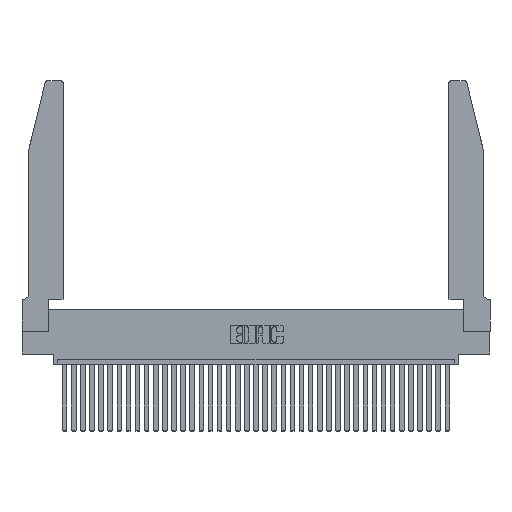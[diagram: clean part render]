
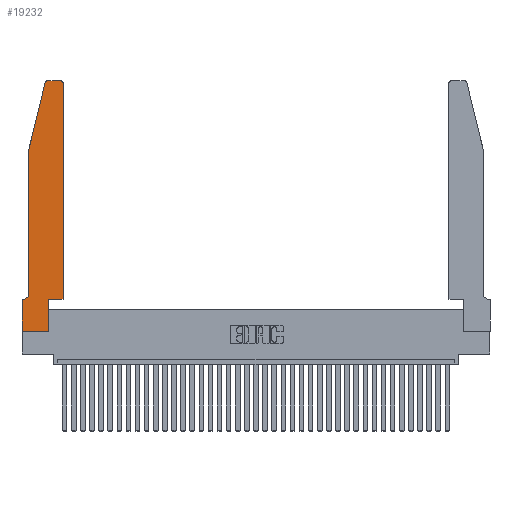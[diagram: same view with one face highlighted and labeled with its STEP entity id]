
A CAD part, top view. The second image highlights one B-rep face of the part: STEP entity #19232.
In plain terms, the highlighted planar face has unit normal (0, 0, 1).
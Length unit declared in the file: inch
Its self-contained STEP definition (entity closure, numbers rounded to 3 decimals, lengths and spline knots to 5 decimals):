
#397 = VERTEX_POINT ( 'NONE', #5148 ) ;
#623 = EDGE_CURVE ( 'NONE', #397, #15735, #32254, .T. ) ;
#2155 = FACE_OUTER_BOUND ( 'NONE', #23706, .T. ) ;
#2720 = DIRECTION ( 'NONE',  ( 0., 0., 1. ) ) ;
#2978 = VERTEX_POINT ( 'NONE', #31135 ) ;
#3154 = EDGE_CURVE ( 'NONE', #24123, #29250, #25392, .T. ) ;
#3217 = ORIENTED_EDGE ( 'NONE', *, *, #3154, .T. ) ;
#3383 = AXIS2_PLACEMENT_3D ( 'NONE', #30027, #23879, #4256 ) ;
#3392 = ORIENTED_EDGE ( 'NONE', *, *, #22904, .T. ) ;
#4256 = DIRECTION ( 'NONE',  ( -1., 0., 0. ) ) ;
#4976 = VECTOR ( 'NONE', #35509, 39.37008 ) ;
#5148 = CARTESIAN_POINT ( 'NONE',  ( 0.25487, 2.72718, 0.37 ) ) ;
#5763 = EDGE_CURVE ( 'NONE', #30272, #30238, #35028, .T. ) ;
#5902 = LINE ( 'NONE', #12907, #19320 ) ;
#6482 = EDGE_CURVE ( 'NONE', #18882, #33333, #8649, .T. ) ;
#7049 = ORIENTED_EDGE ( 'NONE', *, *, #34745, .T. ) ;
#7084 = VERTEX_POINT ( 'NONE', #10803 ) ;
#7914 = CARTESIAN_POINT ( 'NONE',  ( 0.0055, 0.35, 0.37 ) ) ;
#8096 = DIRECTION ( 'NONE',  ( -1., 0., 0. ) ) ;
#8241 = ORIENTED_EDGE ( 'NONE', *, *, #21533, .T. ) ;
#8303 = VECTOR ( 'NONE', #8684, 39.37008 ) ;
#8412 = DIRECTION ( 'NONE',  ( 1., 0., 0. ) ) ;
#8649 = CIRCLE ( 'NONE', #11534, 0.03 ) ;
#8684 = DIRECTION ( 'NONE',  ( 0., 1., 0. ) ) ;
#9523 = VECTOR ( 'NONE', #8096, 39.37008 ) ;
#9739 = CARTESIAN_POINT ( 'NONE',  ( 0.0755, 2., 0.37 ) ) ;
#9882 = DIRECTION ( 'NONE',  ( 0., 0., 1. ) ) ;
#9919 = ORIENTED_EDGE ( 'NONE', *, *, #6482, .T. ) ;
#10495 = EDGE_CURVE ( 'NONE', #2978, #7084, #24878, .T. ) ;
#10749 = CARTESIAN_POINT ( 'NONE',  ( 0.4505, 2.72, 0.37 ) ) ;
#10803 = CARTESIAN_POINT ( 'NONE',  ( 0., 0., 0.37 ) ) ;
#11534 = AXIS2_PLACEMENT_3D ( 'NONE', #13291, #2720, #8412 ) ;
#11841 = CARTESIAN_POINT ( 'NONE',  ( 0., 0.35, 0.37 ) ) ;
#11853 = CARTESIAN_POINT ( 'NONE',  ( 0.0755, 2., 0.37 ) ) ;
#12759 = ORIENTED_EDGE ( 'NONE', *, *, #10495, .T. ) ;
#12907 = CARTESIAN_POINT ( 'NONE',  ( 0., 0., 0.37 ) ) ;
#13291 = CARTESIAN_POINT ( 'NONE',  ( 0.4205, 2.72, 0.37 ) ) ;
#13348 = DIRECTION ( 'NONE',  ( 1., 0., 0. ) ) ;
#13870 = LINE ( 'NONE', #17848, #31223 ) ;
#14028 = EDGE_CURVE ( 'NONE', #29250, #2978, #24976, .T. ) ;
#14050 = CARTESIAN_POINT ( 'NONE',  ( 0., 0., 0.37 ) ) ;
#14905 = DIRECTION ( 'NONE',  ( -0.239, -0.971, 0. ) ) ;
#15240 = ORIENTED_EDGE ( 'NONE', *, *, #5763, .T. ) ;
#15341 = EDGE_CURVE ( 'NONE', #30238, #24344, #17718, .T. ) ;
#15735 = VERTEX_POINT ( 'NONE', #11853 ) ;
#16924 = AXIS2_PLACEMENT_3D ( 'NONE', #32799, #30428, #13348 ) ;
#17277 = VECTOR ( 'NONE', #23079, 39.37008 ) ;
#17515 = VECTOR ( 'NONE', #14905, 39.37008 ) ;
#17718 = LINE ( 'NONE', #23266, #32460 ) ;
#17848 = CARTESIAN_POINT ( 'NONE',  ( 0.4505, 0.35, 0.37 ) ) ;
#17963 = CARTESIAN_POINT ( 'NONE',  ( 0.0755, 2., 0.37 ) ) ;
#17976 = LINE ( 'NONE', #19321, #9523 ) ;
#18375 = ORIENTED_EDGE ( 'NONE', *, *, #14028, .T. ) ;
#18882 = VERTEX_POINT ( 'NONE', #10749 ) ;
#19103 = ORIENTED_EDGE ( 'NONE', *, *, #20784, .T. ) ;
#19232 = ADVANCED_FACE ( 'NONE', ( #2155 ), #26022, .T. ) ;
#19320 = VECTOR ( 'NONE', #21346, 39.37008 ) ;
#19321 = CARTESIAN_POINT ( 'NONE',  ( 0.2605, 2.75, 0.37 ) ) ;
#20571 = CARTESIAN_POINT ( 'NONE',  ( 0.2865, 0.35, 0.37 ) ) ;
#20784 = EDGE_CURVE ( 'NONE', #21955, #397, #35454, .T. ) ;
#20944 = AXIS2_PLACEMENT_3D ( 'NONE', #11841, #9882, #29805 ) ;
#21346 = DIRECTION ( 'NONE',  ( 1., 0., 0. ) ) ;
#21533 = EDGE_CURVE ( 'NONE', #33333, #21955, #17976, .T. ) ;
#21955 = VERTEX_POINT ( 'NONE', #31256 ) ;
#22904 = EDGE_CURVE ( 'NONE', #24344, #18882, #13870, .T. ) ;
#23079 = DIRECTION ( 'NONE',  ( 0., -1., 0. ) ) ;
#23266 = CARTESIAN_POINT ( 'NONE',  ( 0.4505, 0.35, 0.37 ) ) ;
#23706 = EDGE_LOOP ( 'NONE', ( #8241, #19103, #23985, #7049, #3217, #18375, #12759, #33053, #15240, #25656, #3392, #9919 ) ) ;
#23879 = DIRECTION ( 'NONE',  ( 0., 0., -1. ) ) ;
#23985 = ORIENTED_EDGE ( 'NONE', *, *, #623, .T. ) ;
#24123 = VERTEX_POINT ( 'NONE', #36786 ) ;
#24240 = CARTESIAN_POINT ( 'NONE',  ( 0.4205, 2.75, 0.37 ) ) ;
#24344 = VERTEX_POINT ( 'NONE', #29118 ) ;
#24878 = LINE ( 'NONE', #14050, #17277 ) ;
#24976 = LINE ( 'NONE', #35106, #4976 ) ;
#25392 = CIRCLE ( 'NONE', #3383, 0.07 ) ;
#25656 = ORIENTED_EDGE ( 'NONE', *, *, #15341, .T. ) ;
#26022 = PLANE ( 'NONE',  #20944 ) ;
#26284 = DIRECTION ( 'NONE',  ( 0., -1., 0. ) ) ;
#26662 = DIRECTION ( 'NONE',  ( 1., 0., 0. ) ) ;
#26821 = CARTESIAN_POINT ( 'NONE',  ( 0.2865, 0., 0.37 ) ) ;
#28839 = VECTOR ( 'NONE', #26284, 39.37008 ) ;
#29118 = CARTESIAN_POINT ( 'NONE',  ( 0.4505, 0.35, 0.37 ) ) ;
#29250 = VERTEX_POINT ( 'NONE', #7914 ) ;
#29805 = DIRECTION ( 'NONE',  ( 1., 0., 0. ) ) ;
#30027 = CARTESIAN_POINT ( 'NONE',  ( 0.0055, 0.42, 0.37 ) ) ;
#30238 = VERTEX_POINT ( 'NONE', #20571 ) ;
#30272 = VERTEX_POINT ( 'NONE', #26821 ) ;
#30428 = DIRECTION ( 'NONE',  ( 0., 0., 1. ) ) ;
#31135 = CARTESIAN_POINT ( 'NONE',  ( 0., 0.35, 0.37 ) ) ;
#31223 = VECTOR ( 'NONE', #32289, 39.37008 ) ;
#31256 = CARTESIAN_POINT ( 'NONE',  ( 0.284, 2.75, 0.37 ) ) ;
#31336 = CARTESIAN_POINT ( 'NONE',  ( 0.2865, 0.35, 0.37 ) ) ;
#31426 = EDGE_CURVE ( 'NONE', #7084, #30272, #5902, .T. ) ;
#32254 = LINE ( 'NONE', #9739, #17515 ) ;
#32289 = DIRECTION ( 'NONE',  ( 0., 1., 0. ) ) ;
#32460 = VECTOR ( 'NONE', #26662, 39.37008 ) ;
#32799 = CARTESIAN_POINT ( 'NONE',  ( 0.284, 2.72, 0.37 ) ) ;
#33053 = ORIENTED_EDGE ( 'NONE', *, *, #31426, .T. ) ;
#33333 = VERTEX_POINT ( 'NONE', #24240 ) ;
#33787 = LINE ( 'NONE', #17963, #28839 ) ;
#34745 = EDGE_CURVE ( 'NONE', #15735, #24123, #33787, .T. ) ;
#35028 = LINE ( 'NONE', #31336, #8303 ) ;
#35106 = CARTESIAN_POINT ( 'NONE',  ( 0.0755, 0.35, 0.37 ) ) ;
#35454 = CIRCLE ( 'NONE', #16924, 0.03 ) ;
#35509 = DIRECTION ( 'NONE',  ( -1., 0., 0. ) ) ;
#36786 = CARTESIAN_POINT ( 'NONE',  ( 0.0755, 0.42, 0.37 ) ) ;
